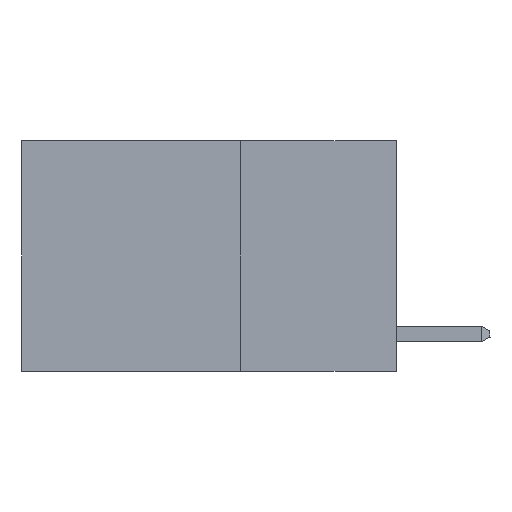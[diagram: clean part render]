
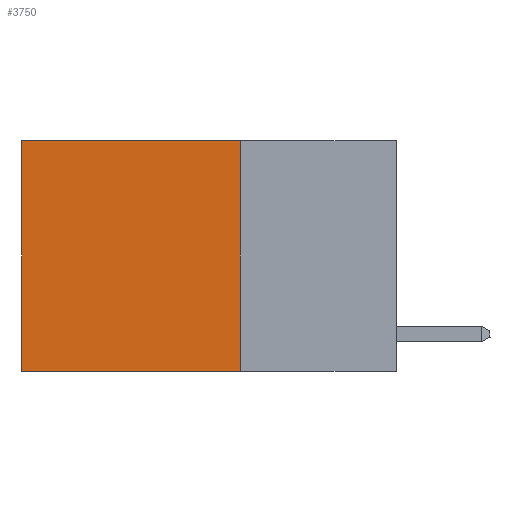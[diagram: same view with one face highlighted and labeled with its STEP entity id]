
A CAD part, left-side view. The second image highlights one B-rep face of the part: STEP entity #3750.
In plain terms, the highlighted planar face has unit normal (-1, 0, 0).
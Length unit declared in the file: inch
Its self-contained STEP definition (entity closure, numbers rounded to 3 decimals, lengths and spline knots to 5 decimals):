
#743 = FACE_OUTER_BOUND ( 'NONE', #14304, .T. ) ;
#1490 = EDGE_CURVE ( 'NONE', #19474, #10102, #9486, .T. ) ;
#1899 = CARTESIAN_POINT ( 'NONE',  ( 0.2625, 0.6, 0. ) ) ;
#2096 = VECTOR ( 'NONE', #6832, 39.37008 ) ;
#3288 = EDGE_CURVE ( 'NONE', #15713, #19474, #18145, .T. ) ;
#3750 = ADVANCED_FACE ( 'NONE', ( #743 ), #5445, .F. ) ;
#3952 = LINE ( 'NONE', #14573, #11704 ) ;
#4182 = ORIENTED_EDGE ( 'NONE', *, *, #8100, .F. ) ;
#5026 = DIRECTION ( 'NONE',  ( 0., 1., 0. ) ) ;
#5445 = PLANE ( 'NONE',  #6466 ) ;
#5546 = DIRECTION ( 'NONE',  ( 0., 0., -1. ) ) ;
#6451 = CARTESIAN_POINT ( 'NONE',  ( 0.2625, 0.6, 0. ) ) ;
#6466 = AXIS2_PLACEMENT_3D ( 'NONE', #8804, #7005, #5546 ) ;
#6832 = DIRECTION ( 'NONE',  ( 0., 1., 0. ) ) ;
#7005 = DIRECTION ( 'NONE',  ( 1., 0., 0. ) ) ;
#7861 = DIRECTION ( 'NONE',  ( 0., 0., -1. ) ) ;
#8100 = EDGE_CURVE ( 'NONE', #15713, #13815, #13836, .T. ) ;
#8804 = CARTESIAN_POINT ( 'NONE',  ( 0.2625, 0.25, 0. ) ) ;
#8883 = CARTESIAN_POINT ( 'NONE',  ( 0.2625, 0.25, -0.37 ) ) ;
#9486 = LINE ( 'NONE', #6451, #16930 ) ;
#9490 = ORIENTED_EDGE ( 'NONE', *, *, #1490, .T. ) ;
#9494 = VECTOR ( 'NONE', #7861, 39.37008 ) ;
#10102 = VERTEX_POINT ( 'NONE', #13656 ) ;
#11368 = DIRECTION ( 'NONE',  ( 0., 0., -1. ) ) ;
#11704 = VECTOR ( 'NONE', #5026, 39.37008 ) ;
#12607 = ORIENTED_EDGE ( 'NONE', *, *, #18144, .F. ) ;
#13656 = CARTESIAN_POINT ( 'NONE',  ( 0.2625, 0.6, -0.37 ) ) ;
#13786 = ORIENTED_EDGE ( 'NONE', *, *, #3288, .T. ) ;
#13815 = VERTEX_POINT ( 'NONE', #8883 ) ;
#13836 = LINE ( 'NONE', #20325, #9494 ) ;
#14304 = EDGE_LOOP ( 'NONE', ( #9490, #12607, #4182, #13786 ) ) ;
#14573 = CARTESIAN_POINT ( 'NONE',  ( 0.2625, 0.25, -0.37 ) ) ;
#14990 = CARTESIAN_POINT ( 'NONE',  ( 0.2625, 0.25, 0. ) ) ;
#15713 = VERTEX_POINT ( 'NONE', #15866 ) ;
#15866 = CARTESIAN_POINT ( 'NONE',  ( 0.2625, 0.25, 0. ) ) ;
#16930 = VECTOR ( 'NONE', #11368, 39.37008 ) ;
#18144 = EDGE_CURVE ( 'NONE', #13815, #10102, #3952, .T. ) ;
#18145 = LINE ( 'NONE', #14990, #2096 ) ;
#19474 = VERTEX_POINT ( 'NONE', #1899 ) ;
#20325 = CARTESIAN_POINT ( 'NONE',  ( 0.2625, 0.25, 0. ) ) ;
